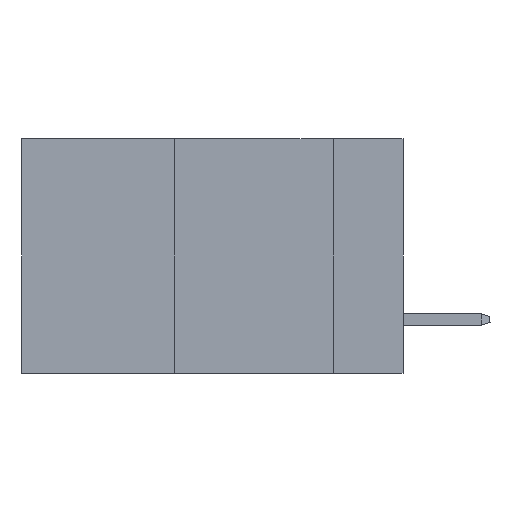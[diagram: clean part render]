
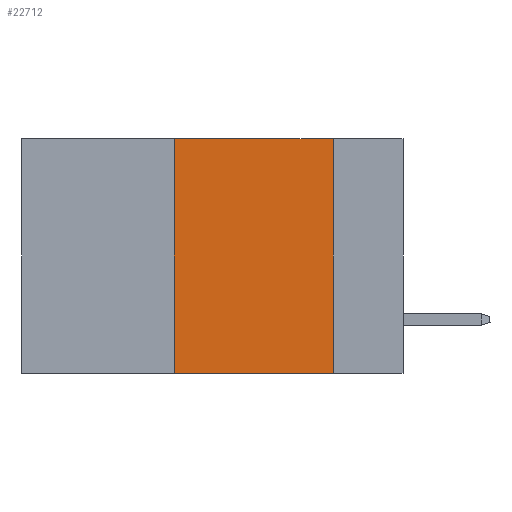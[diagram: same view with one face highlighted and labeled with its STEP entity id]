
A CAD part, left-side view. The second image highlights one B-rep face of the part: STEP entity #22712.
In plain terms, the highlighted planar face has unit normal (-1, 0, 0).
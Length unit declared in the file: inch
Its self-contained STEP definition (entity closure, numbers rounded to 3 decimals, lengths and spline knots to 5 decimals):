
#46 = CARTESIAN_POINT ( 'NONE',  ( 0., 0.36, 0. ) ) ;
#1708 = EDGE_CURVE ( 'NONE', #16631, #20317, #19915, .T. ) ;
#3726 = LINE ( 'NONE', #35527, #51215 ) ;
#5292 = VECTOR ( 'NONE', #27993, 39.37008 ) ;
#5644 = DIRECTION ( 'NONE',  ( 0., 0., -1. ) ) ;
#6151 = PLANE ( 'NONE',  #49434 ) ;
#9529 = VERTEX_POINT ( 'NONE', #41160 ) ;
#9532 = DIRECTION ( 'NONE',  ( 0., -1., 0. ) ) ;
#10060 = DIRECTION ( 'NONE',  ( 0., 0., -1. ) ) ;
#12397 = LINE ( 'NONE', #44223, #43472 ) ;
#14573 = EDGE_LOOP ( 'NONE', ( #20216, #45380, #41315, #48242 ) ) ;
#14734 = FACE_OUTER_BOUND ( 'NONE', #14573, .T. ) ;
#16631 = VERTEX_POINT ( 'NONE', #46 ) ;
#17984 = VECTOR ( 'NONE', #5644, 39.37008 ) ;
#18129 = CARTESIAN_POINT ( 'NONE',  ( 0., 0.6, 0. ) ) ;
#19915 = LINE ( 'NONE', #47828, #5292 ) ;
#20216 = ORIENTED_EDGE ( 'NONE', *, *, #27616, .F. ) ;
#20317 = VERTEX_POINT ( 'NONE', #41568 ) ;
#20408 = DIRECTION ( 'NONE',  ( 0., 0., 1. ) ) ;
#22712 = ADVANCED_FACE ( 'NONE', ( #14734 ), #6151, .F. ) ;
#27616 = EDGE_CURVE ( 'NONE', #20317, #9529, #46055, .T. ) ;
#27993 = DIRECTION ( 'NONE',  ( 0., -1., 0. ) ) ;
#35527 = CARTESIAN_POINT ( 'NONE',  ( 0., 0.36, 0. ) ) ;
#36250 = EDGE_CURVE ( 'NONE', #47255, #9529, #12397, .T. ) ;
#38918 = CARTESIAN_POINT ( 'NONE',  ( 0., 0.36, -0.37 ) ) ;
#41160 = CARTESIAN_POINT ( 'NONE',  ( 0., 0.11, -0.37 ) ) ;
#41225 = EDGE_CURVE ( 'NONE', #47255, #16631, #3726, .T. ) ;
#41315 = ORIENTED_EDGE ( 'NONE', *, *, #41225, .F. ) ;
#41568 = CARTESIAN_POINT ( 'NONE',  ( 0., 0.11, 0. ) ) ;
#43472 = VECTOR ( 'NONE', #9532, 39.37008 ) ;
#44223 = CARTESIAN_POINT ( 'NONE',  ( 0., 0.6, -0.37 ) ) ;
#45380 = ORIENTED_EDGE ( 'NONE', *, *, #1708, .F. ) ;
#45783 = DIRECTION ( 'NONE',  ( 1., 0., 0. ) ) ;
#45790 = CARTESIAN_POINT ( 'NONE',  ( 0., 0.11, 0. ) ) ;
#46055 = LINE ( 'NONE', #45790, #17984 ) ;
#47255 = VERTEX_POINT ( 'NONE', #38918 ) ;
#47828 = CARTESIAN_POINT ( 'NONE',  ( 0., 0.6, 0. ) ) ;
#48242 = ORIENTED_EDGE ( 'NONE', *, *, #36250, .T. ) ;
#49434 = AXIS2_PLACEMENT_3D ( 'NONE', #18129, #45783, #10060 ) ;
#51215 = VECTOR ( 'NONE', #20408, 39.37008 ) ;
